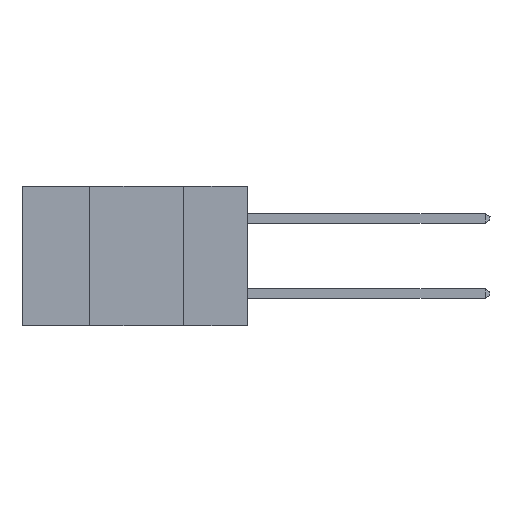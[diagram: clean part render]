
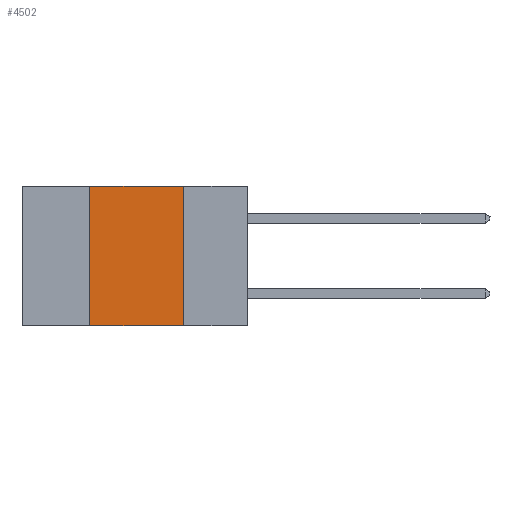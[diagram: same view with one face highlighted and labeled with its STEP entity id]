
A CAD part, left-side view. The second image highlights one B-rep face of the part: STEP entity #4502.
In plain terms, the highlighted planar face has unit normal (-1, 0, 0).
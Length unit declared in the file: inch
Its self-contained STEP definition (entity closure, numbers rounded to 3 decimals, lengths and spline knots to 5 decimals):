
#179 = DIRECTION ( 'NONE',  ( 0., 0., 1. ) ) ;
#657 = CARTESIAN_POINT ( 'NONE',  ( 0., 0.42, 0. ) ) ;
#2791 = VERTEX_POINT ( 'NONE', #7751 ) ;
#3721 = DIRECTION ( 'NONE',  ( 0., -1., 0. ) ) ;
#3817 = CARTESIAN_POINT ( 'NONE',  ( 0., 0.42, -0.37 ) ) ;
#3841 = EDGE_CURVE ( 'NONE', #8881, #15487, #11599, .T. ) ;
#4336 = LINE ( 'NONE', #5504, #11067 ) ;
#4502 = ADVANCED_FACE ( 'NONE', ( #11052 ), #15169, .F. ) ;
#4733 = EDGE_LOOP ( 'NONE', ( #15351, #15621, #8475, #12431 ) ) ;
#5161 = DIRECTION ( 'NONE',  ( 0., 0., -1. ) ) ;
#5504 = CARTESIAN_POINT ( 'NONE',  ( 0., 0.6, 0. ) ) ;
#6596 = DIRECTION ( 'NONE',  ( 0., -1., 0. ) ) ;
#6687 = CARTESIAN_POINT ( 'NONE',  ( 0., 0.42, -0.37 ) ) ;
#7252 = CARTESIAN_POINT ( 'NONE',  ( 0., 0.17, -0.37 ) ) ;
#7680 = AXIS2_PLACEMENT_3D ( 'NONE', #11290, #8771, #12728 ) ;
#7751 = CARTESIAN_POINT ( 'NONE',  ( 0., 0.17, 0. ) ) ;
#8475 = ORIENTED_EDGE ( 'NONE', *, *, #11286, .F. ) ;
#8574 = EDGE_CURVE ( 'NONE', #10103, #2791, #4336, .T. ) ;
#8771 = DIRECTION ( 'NONE',  ( 1., 0., 0. ) ) ;
#8881 = VERTEX_POINT ( 'NONE', #3817 ) ;
#9024 = CARTESIAN_POINT ( 'NONE',  ( 0., 0.17, -0.37 ) ) ;
#10103 = VERTEX_POINT ( 'NONE', #657 ) ;
#10344 = CARTESIAN_POINT ( 'NONE',  ( 0., 0.6, -0.37 ) ) ;
#10539 = VECTOR ( 'NONE', #179, 39.37008 ) ;
#11052 = FACE_OUTER_BOUND ( 'NONE', #4733, .T. ) ;
#11067 = VECTOR ( 'NONE', #6596, 39.37008 ) ;
#11286 = EDGE_CURVE ( 'NONE', #8881, #10103, #12922, .T. ) ;
#11290 = CARTESIAN_POINT ( 'NONE',  ( 0., 0.6, 0. ) ) ;
#11599 = LINE ( 'NONE', #10344, #12479 ) ;
#11630 = EDGE_CURVE ( 'NONE', #2791, #15487, #13137, .T. ) ;
#12431 = ORIENTED_EDGE ( 'NONE', *, *, #3841, .T. ) ;
#12479 = VECTOR ( 'NONE', #3721, 39.37008 ) ;
#12728 = DIRECTION ( 'NONE',  ( 0., 0., -1. ) ) ;
#12922 = LINE ( 'NONE', #6687, #10539 ) ;
#13137 = LINE ( 'NONE', #9024, #14842 ) ;
#14842 = VECTOR ( 'NONE', #5161, 39.37008 ) ;
#15169 = PLANE ( 'NONE',  #7680 ) ;
#15351 = ORIENTED_EDGE ( 'NONE', *, *, #11630, .F. ) ;
#15487 = VERTEX_POINT ( 'NONE', #7252 ) ;
#15621 = ORIENTED_EDGE ( 'NONE', *, *, #8574, .F. ) ;
